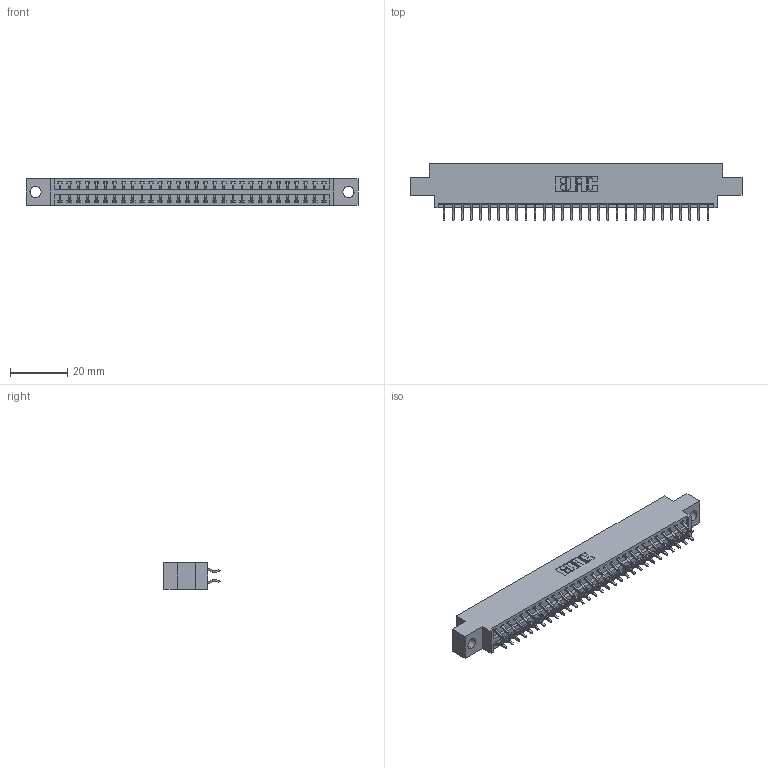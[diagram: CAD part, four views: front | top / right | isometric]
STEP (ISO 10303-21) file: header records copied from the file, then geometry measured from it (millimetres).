
FILE_DESCRIPTION (( 'STEP AP203' ), '1' );
FILE_NAME ('346-060-556-804.STEP', '2022-05-21T12:08:26', ( '' ), ( '' ), 'SwSTEP 2.0', 'SolidWorks 2020', '' );
FILE_SCHEMA (( 'CONFIG_CONTROL_DESIGN' ));
Length unit declared in the file: inch
Products named in the file (3): 345-292-001_556 Tail; 346 Part_0.170 Offset - 0.156 Dia-TH; 346-060-556-804
Assembly tree (61 placements, depth 2):
  346-060-556-804
    346 Part_0.170 Offset - 0.156 Dia-TH
    345-292-001_556 Tail  x60
Bounding box: 115.82 x 19.57 x 9.4 mm (x, y, z)
Volume: 10938.1 mm3; surface area: 14818.4 mm2
Topology: 61 solids, 61 shells, 3620 faces, 10757 edges, 7090 vertices
Faces by surface type: plane 2434, cylinder 1186
Entity records: 21965 total; most frequent: CARTESIAN_POINT 3658, ORIENTED_EDGE 3578, DIRECTION 3261, EDGE_CURVE 1789, VECTOR 1529, LINE 1529, VERTEX_POINT 1190, AXIS2_PLACEMENT_3D 866
